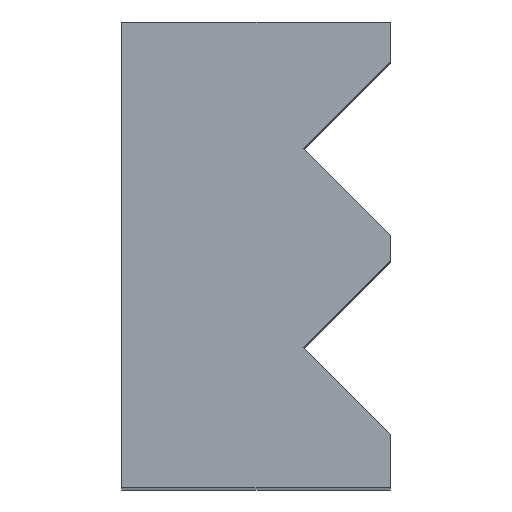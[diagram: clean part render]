
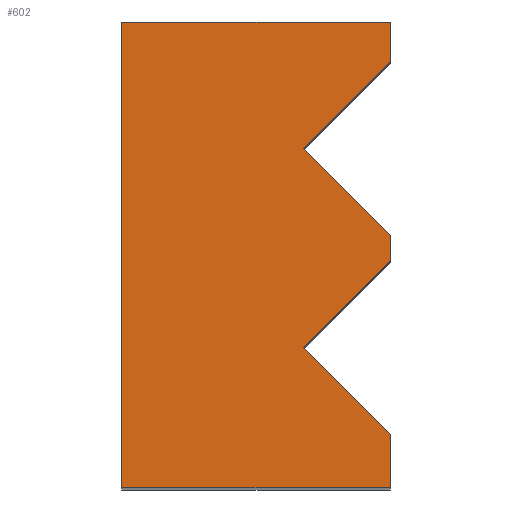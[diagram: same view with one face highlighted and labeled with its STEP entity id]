
A CAD part, top view. The second image highlights one B-rep face of the part: STEP entity #602.
In plain terms, the highlighted planar face has unit normal (0, 0, 1).
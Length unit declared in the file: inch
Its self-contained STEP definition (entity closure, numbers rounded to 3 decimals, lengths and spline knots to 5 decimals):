
#2 = VECTOR ( 'NONE', #619, 39.37008 ) ;
#5 = FACE_OUTER_BOUND ( 'NONE', #119, .T. ) ;
#10 = VERTEX_POINT ( 'NONE', #537 ) ;
#13 = VERTEX_POINT ( 'NONE', #484 ) ;
#19 = VERTEX_POINT ( 'NONE', #184 ) ;
#20 = LINE ( 'NONE', #529, #154 ) ;
#46 = ORIENTED_EDGE ( 'NONE', *, *, #414, .T. ) ;
#49 = VECTOR ( 'NONE', #151, 39.37008 ) ;
#69 = ORIENTED_EDGE ( 'NONE', *, *, #486, .T. ) ;
#76 = EDGE_CURVE ( 'NONE', #153, #704, #483, .T. ) ;
#93 = EDGE_CURVE ( 'NONE', #10, #474, #168, .T. ) ;
#108 = EDGE_CURVE ( 'NONE', #427, #421, #590, .T. ) ;
#110 = CARTESIAN_POINT ( 'NONE',  ( -0.428, 0.152, 1.25 ) ) ;
#111 = VECTOR ( 'NONE', #566, 39.37008 ) ;
#118 = DIRECTION ( 'NONE',  ( 0., -1., 0. ) ) ;
#119 = EDGE_LOOP ( 'NONE', ( #46, #145, #604, #424, #344, #507, #69, #530, #366, #142 ) ) ;
#139 = CARTESIAN_POINT ( 'NONE',  ( -0.625, 0., 1.25 ) ) ;
#141 = DIRECTION ( 'NONE',  ( 0.707, 0.707, 0. ) ) ;
#142 = ORIENTED_EDGE ( 'NONE', *, *, #93, .T. ) ;
#145 = ORIENTED_EDGE ( 'NONE', *, *, #600, .F. ) ;
#151 = DIRECTION ( 'NONE',  ( 0., -1., 0. ) ) ;
#152 = LINE ( 'NONE', #210, #2 ) ;
#153 = VERTEX_POINT ( 'NONE', #663 ) ;
#154 = VECTOR ( 'NONE', #118, 39.37008 ) ;
#160 = CARTESIAN_POINT ( 'NONE',  ( -0.428, 0.152, 1.25 ) ) ;
#168 = LINE ( 'NONE', #139, #632 ) ;
#178 = CARTESIAN_POINT ( 'NONE',  ( -0.625, 0.505, 1.25 ) ) ;
#181 = VECTOR ( 'NONE', #713, 39.37008 ) ;
#184 = CARTESIAN_POINT ( 'NONE',  ( -0.428, 0.368, 1.25 ) ) ;
#196 = DIRECTION ( 'NONE',  ( 0., -1., 0. ) ) ;
#210 = CARTESIAN_POINT ( 'NONE',  ( -0.3085, 0.505, 1.25 ) ) ;
#218 = EDGE_CURVE ( 'NONE', #153, #10, #152, .T. ) ;
#233 = DIRECTION ( 'NONE',  ( -0.707, 0.707, 0. ) ) ;
#241 = PLANE ( 'NONE',  #450 ) ;
#246 = VECTOR ( 'NONE', #233, 39.37008 ) ;
#264 = CARTESIAN_POINT ( 'NONE',  ( -0.3335, 0.4625, 1.25 ) ) ;
#266 = LINE ( 'NONE', #110, #246 ) ;
#269 = EDGE_CURVE ( 'NONE', #338, #19, #582, .T. ) ;
#279 = CARTESIAN_POINT ( 'NONE',  ( -0.3335, 0.0575, 1.25 ) ) ;
#305 = DIRECTION ( 'NONE',  ( 0., 0., -1. ) ) ;
#306 = LINE ( 'NONE', #520, #723 ) ;
#318 = CARTESIAN_POINT ( 'NONE',  ( -0.3335, 0.505, 1.25 ) ) ;
#337 = CARTESIAN_POINT ( 'NONE',  ( -0.3335, 0.2465, 1.25 ) ) ;
#338 = VERTEX_POINT ( 'NONE', #403 ) ;
#344 = ORIENTED_EDGE ( 'NONE', *, *, #712, .F. ) ;
#360 = LINE ( 'NONE', #502, #49 ) ;
#366 = ORIENTED_EDGE ( 'NONE', *, *, #218, .T. ) ;
#391 = VERTEX_POINT ( 'NONE', #279 ) ;
#403 = CARTESIAN_POINT ( 'NONE',  ( -0.3335, 0.2735, 1.25 ) ) ;
#414 = EDGE_CURVE ( 'NONE', #474, #13, #641, .T. ) ;
#421 = VERTEX_POINT ( 'NONE', #337 ) ;
#424 = ORIENTED_EDGE ( 'NONE', *, *, #108, .T. ) ;
#427 = VERTEX_POINT ( 'NONE', #160 ) ;
#439 = VECTOR ( 'NONE', #141, 39.37008 ) ;
#450 = AXIS2_PLACEMENT_3D ( 'NONE', #178, #305, #699 ) ;
#474 = VERTEX_POINT ( 'NONE', #574 ) ;
#483 = LINE ( 'NONE', #318, #181 ) ;
#484 = CARTESIAN_POINT ( 'NONE',  ( -0.3335, 0., 1.25 ) ) ;
#486 = EDGE_CURVE ( 'NONE', #19, #704, #306, .T. ) ;
#502 = CARTESIAN_POINT ( 'NONE',  ( -0.3335, 0.505, 1.25 ) ) ;
#507 = ORIENTED_EDGE ( 'NONE', *, *, #269, .T. ) ;
#509 = CARTESIAN_POINT ( 'NONE',  ( -0.428, 0.368, 1.25 ) ) ;
#520 = CARTESIAN_POINT ( 'NONE',  ( -0.32, 0.476, 1.25 ) ) ;
#526 = EDGE_CURVE ( 'NONE', #391, #427, #266, .T. ) ;
#529 = CARTESIAN_POINT ( 'NONE',  ( -0.3335, 0.505, 1.25 ) ) ;
#530 = ORIENTED_EDGE ( 'NONE', *, *, #76, .F. ) ;
#537 = CARTESIAN_POINT ( 'NONE',  ( -0.625, 0.505, 1.25 ) ) ;
#566 = DIRECTION ( 'NONE',  ( -0.707, 0.707, 0. ) ) ;
#567 = DIRECTION ( 'NONE',  ( 1., 0., 0. ) ) ;
#574 = CARTESIAN_POINT ( 'NONE',  ( -0.625, 0., 1.25 ) ) ;
#582 = LINE ( 'NONE', #509, #111 ) ;
#590 = LINE ( 'NONE', #606, #439 ) ;
#600 = EDGE_CURVE ( 'NONE', #391, #13, #20, .T. ) ;
#602 = ADVANCED_FACE ( 'NONE', ( #5 ), #241, .F. ) ;
#604 = ORIENTED_EDGE ( 'NONE', *, *, #526, .T. ) ;
#606 = CARTESIAN_POINT ( 'NONE',  ( -0.32, 0.26, 1.25 ) ) ;
#612 = VECTOR ( 'NONE', #567, 39.37008 ) ;
#619 = DIRECTION ( 'NONE',  ( -1., 0., 0. ) ) ;
#631 = DIRECTION ( 'NONE',  ( 0.707, 0.707, 0. ) ) ;
#632 = VECTOR ( 'NONE', #196, 39.37008 ) ;
#641 = LINE ( 'NONE', #738, #612 ) ;
#663 = CARTESIAN_POINT ( 'NONE',  ( -0.3335, 0.505, 1.25 ) ) ;
#699 = DIRECTION ( 'NONE',  ( -1., 0., 0. ) ) ;
#704 = VERTEX_POINT ( 'NONE', #264 ) ;
#712 = EDGE_CURVE ( 'NONE', #338, #421, #360, .T. ) ;
#713 = DIRECTION ( 'NONE',  ( 0., -1., 0. ) ) ;
#723 = VECTOR ( 'NONE', #631, 39.37008 ) ;
#738 = CARTESIAN_POINT ( 'NONE',  ( -0.32, 0., 1.25 ) ) ;
